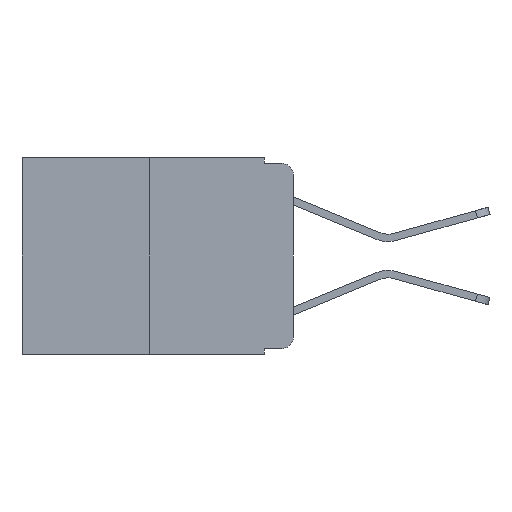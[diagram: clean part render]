
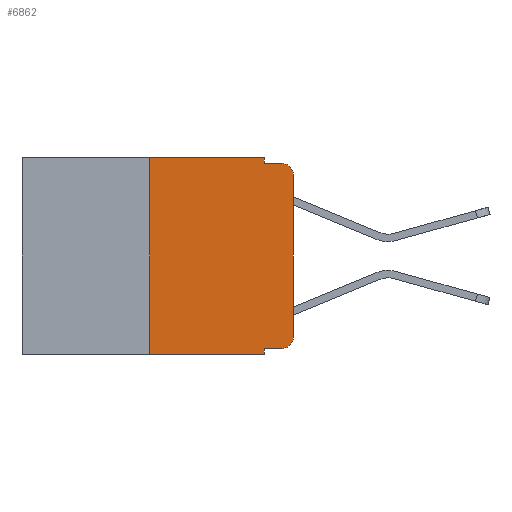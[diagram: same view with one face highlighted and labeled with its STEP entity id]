
A CAD part, left-side view. The second image highlights one B-rep face of the part: STEP entity #6862.
In plain terms, the highlighted planar face has unit normal (-1, 0, 0).
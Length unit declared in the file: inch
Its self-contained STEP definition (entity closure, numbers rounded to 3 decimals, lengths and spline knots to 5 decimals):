
#42 = CARTESIAN_POINT ( 'NONE',  ( 0., 0.473, 0. ) ) ;
#237 = LINE ( 'NONE', #42, #9769 ) ;
#466 = EDGE_CURVE ( 'NONE', #7961, #7943, #237, .T. ) ;
#531 = CIRCLE ( 'NONE', #9288, 0.02 ) ;
#609 = VERTEX_POINT ( 'NONE', #10784 ) ;
#1004 = DIRECTION ( 'NONE',  ( -1., 0., 0. ) ) ;
#1028 = ORIENTED_EDGE ( 'NONE', *, *, #8961, .F. ) ;
#1124 = LINE ( 'NONE', #10419, #3723 ) ;
#1149 = CARTESIAN_POINT ( 'NONE',  ( 0., 0.051, -0.01 ) ) ;
#1156 = EDGE_LOOP ( 'NONE', ( #8014, #9986, #4798, #6934, #8945, #8682, #6093, #1028, #5814, #7602 ) ) ;
#1363 = LINE ( 'NONE', #9339, #3656 ) ;
#1607 = VERTEX_POINT ( 'NONE', #4604 ) ;
#1609 = VERTEX_POINT ( 'NONE', #9703 ) ;
#1791 = CARTESIAN_POINT ( 'NONE',  ( 0., 0.051, 0. ) ) ;
#2003 = VECTOR ( 'NONE', #5891, 39.37008 ) ;
#2432 = CARTESIAN_POINT ( 'NONE',  ( 0., 0.02, -0.333 ) ) ;
#2476 = VECTOR ( 'NONE', #8220, 39.37008 ) ;
#2575 = PLANE ( 'NONE',  #9984 ) ;
#2612 = VERTEX_POINT ( 'NONE', #2432 ) ;
#2671 = VERTEX_POINT ( 'NONE', #10093 ) ;
#3656 = VECTOR ( 'NONE', #10174, 39.37008 ) ;
#3712 = VECTOR ( 'NONE', #9118, 39.37008 ) ;
#3723 = VECTOR ( 'NONE', #4339, 39.37008 ) ;
#3814 = AXIS2_PLACEMENT_3D ( 'NONE', #6671, #1004, #7549 ) ;
#3817 = CARTESIAN_POINT ( 'NONE',  ( 0., 0.051, 0. ) ) ;
#3871 = DIRECTION ( 'NONE',  ( -1., 0., 0. ) ) ;
#3872 = CARTESIAN_POINT ( 'NONE',  ( 0., 0., -0.03 ) ) ;
#4075 = LINE ( 'NONE', #1791, #10751 ) ;
#4339 = DIRECTION ( 'NONE',  ( 0., 0., 1. ) ) ;
#4604 = CARTESIAN_POINT ( 'NONE',  ( 0., 0.25, -0.343 ) ) ;
#4628 = DIRECTION ( 'NONE',  ( 0., 0., -1. ) ) ;
#4798 = ORIENTED_EDGE ( 'NONE', *, *, #7114, .F. ) ;
#4980 = CARTESIAN_POINT ( 'NONE',  ( 0., 0.02, -0.01 ) ) ;
#5388 = VERTEX_POINT ( 'NONE', #8854 ) ;
#5408 = CARTESIAN_POINT ( 'NONE',  ( 0., 0.473, 0. ) ) ;
#5617 = EDGE_CURVE ( 'NONE', #7943, #1609, #8731, .T. ) ;
#5736 = CARTESIAN_POINT ( 'NONE',  ( 0., 0.051, 0. ) ) ;
#5814 = ORIENTED_EDGE ( 'NONE', *, *, #10215, .T. ) ;
#5891 = DIRECTION ( 'NONE',  ( 0., -1., 0. ) ) ;
#6093 = ORIENTED_EDGE ( 'NONE', *, *, #8709, .T. ) ;
#6285 = EDGE_CURVE ( 'NONE', #609, #10240, #7378, .T. ) ;
#6319 = DIRECTION ( 'NONE',  ( 0., 0., -1. ) ) ;
#6463 = LINE ( 'NONE', #10812, #10718 ) ;
#6671 = CARTESIAN_POINT ( 'NONE',  ( 0., 0.02, -0.03 ) ) ;
#6862 = ADVANCED_FACE ( 'NONE', ( #9089 ), #2575, .F. ) ;
#6934 = ORIENTED_EDGE ( 'NONE', *, *, #5617, .F. ) ;
#7114 = EDGE_CURVE ( 'NONE', #1609, #9167, #11432, .T. ) ;
#7367 = CARTESIAN_POINT ( 'NONE',  ( 0., 0., 0. ) ) ;
#7378 = LINE ( 'NONE', #7367, #2476 ) ;
#7549 = DIRECTION ( 'NONE',  ( 0., 0., -1. ) ) ;
#7602 = ORIENTED_EDGE ( 'NONE', *, *, #8560, .T. ) ;
#7943 = VERTEX_POINT ( 'NONE', #5736 ) ;
#7961 = VERTEX_POINT ( 'NONE', #8370 ) ;
#7976 = EDGE_CURVE ( 'NONE', #10240, #9167, #11034, .T. ) ;
#8014 = ORIENTED_EDGE ( 'NONE', *, *, #6285, .T. ) ;
#8220 = DIRECTION ( 'NONE',  ( 0., 0., 1. ) ) ;
#8370 = CARTESIAN_POINT ( 'NONE',  ( 0., 0.25, 0. ) ) ;
#8560 = EDGE_CURVE ( 'NONE', #2612, #609, #531, .T. ) ;
#8682 = ORIENTED_EDGE ( 'NONE', *, *, #11350, .F. ) ;
#8709 = EDGE_CURVE ( 'NONE', #1607, #2671, #1363, .T. ) ;
#8731 = LINE ( 'NONE', #3817, #3712 ) ;
#8854 = CARTESIAN_POINT ( 'NONE',  ( 0., 0.051, -0.333 ) ) ;
#8945 = ORIENTED_EDGE ( 'NONE', *, *, #466, .F. ) ;
#8961 = EDGE_CURVE ( 'NONE', #5388, #2671, #4075, .T. ) ;
#9089 = FACE_OUTER_BOUND ( 'NONE', #1156, .T. ) ;
#9118 = DIRECTION ( 'NONE',  ( 0., 0., -1. ) ) ;
#9164 = CARTESIAN_POINT ( 'NONE',  ( 0., 0.02, -0.313 ) ) ;
#9167 = VERTEX_POINT ( 'NONE', #4980 ) ;
#9288 = AXIS2_PLACEMENT_3D ( 'NONE', #9164, #3871, #10000 ) ;
#9339 = CARTESIAN_POINT ( 'NONE',  ( 0., 0.473, -0.343 ) ) ;
#9703 = CARTESIAN_POINT ( 'NONE',  ( 0., 0.051, -0.01 ) ) ;
#9769 = VECTOR ( 'NONE', #11662, 39.37008 ) ;
#9969 = DIRECTION ( 'NONE',  ( 0., -1., 0. ) ) ;
#9984 = AXIS2_PLACEMENT_3D ( 'NONE', #5408, #11400, #6319 ) ;
#9986 = ORIENTED_EDGE ( 'NONE', *, *, #7976, .T. ) ;
#10000 = DIRECTION ( 'NONE',  ( 0., 0., -1. ) ) ;
#10093 = CARTESIAN_POINT ( 'NONE',  ( 0., 0.051, -0.343 ) ) ;
#10174 = DIRECTION ( 'NONE',  ( 0., -1., 0. ) ) ;
#10215 = EDGE_CURVE ( 'NONE', #5388, #2612, #6463, .T. ) ;
#10240 = VERTEX_POINT ( 'NONE', #3872 ) ;
#10419 = CARTESIAN_POINT ( 'NONE',  ( 0., 0.25, 0. ) ) ;
#10718 = VECTOR ( 'NONE', #9969, 39.37008 ) ;
#10751 = VECTOR ( 'NONE', #4628, 39.37008 ) ;
#10784 = CARTESIAN_POINT ( 'NONE',  ( 0., 0., -0.313 ) ) ;
#10812 = CARTESIAN_POINT ( 'NONE',  ( 0., 0.051, -0.333 ) ) ;
#11034 = CIRCLE ( 'NONE', #3814, 0.02 ) ;
#11350 = EDGE_CURVE ( 'NONE', #1607, #7961, #1124, .T. ) ;
#11400 = DIRECTION ( 'NONE',  ( 1., 0., 0. ) ) ;
#11432 = LINE ( 'NONE', #1149, #2003 ) ;
#11662 = DIRECTION ( 'NONE',  ( 0., -1., 0. ) ) ;
